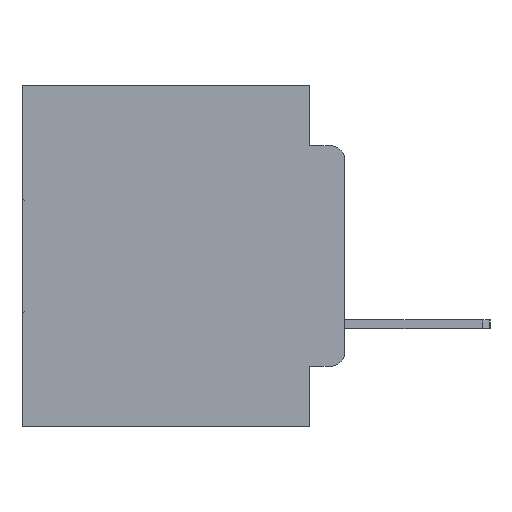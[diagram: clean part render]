
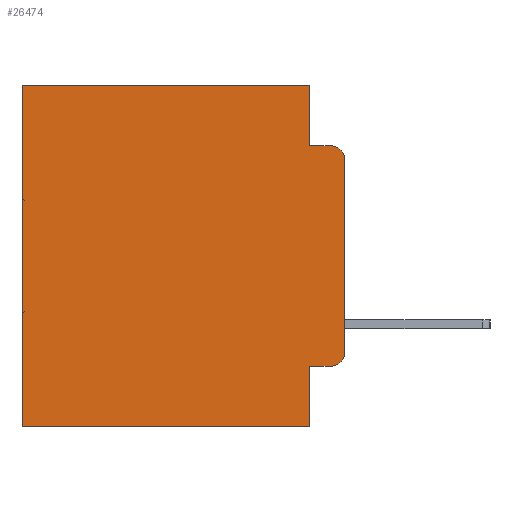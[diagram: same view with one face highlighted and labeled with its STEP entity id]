
A CAD part, left-side view. The second image highlights one B-rep face of the part: STEP entity #26474.
In plain terms, the highlighted planar face has unit normal (-1, 0, 0).
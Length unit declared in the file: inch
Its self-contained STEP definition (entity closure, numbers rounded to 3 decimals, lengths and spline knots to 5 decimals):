
#558 = FACE_OUTER_BOUND ( 'NONE', #12549, .T. ) ;
#746 = EDGE_CURVE ( 'NONE', #23154, #11562, #28423, .T. ) ;
#1446 = EDGE_CURVE ( 'NONE', #12191, #9325, #27314, .T. ) ;
#1615 = ORIENTED_EDGE ( 'NONE', *, *, #20073, .T. ) ;
#2730 = DIRECTION ( 'NONE',  ( 1., 0., 0. ) ) ;
#2898 = VECTOR ( 'NONE', #12194, 39.37008 ) ;
#3358 = CARTESIAN_POINT ( 'NONE',  ( 0.298, 0.02, -0.0885 ) ) ;
#3398 = CARTESIAN_POINT ( 'NONE',  ( 0.298, 0., -0.1085 ) ) ;
#3551 = VECTOR ( 'NONE', #27947, 39.37008 ) ;
#4354 = DIRECTION ( 'NONE',  ( 0., 1., 0. ) ) ;
#4423 = ORIENTED_EDGE ( 'NONE', *, *, #24221, .F. ) ;
#4922 = VERTEX_POINT ( 'NONE', #20242 ) ;
#4966 = ORIENTED_EDGE ( 'NONE', *, *, #13265, .T. ) ;
#5223 = CARTESIAN_POINT ( 'NONE',  ( 0.298, 0.473, 0. ) ) ;
#5248 = DIRECTION ( 'NONE',  ( 0., 0., -1. ) ) ;
#6202 = VERTEX_POINT ( 'NONE', #22765 ) ;
#6995 = EDGE_CURVE ( 'NONE', #4922, #6202, #16270, .T. ) ;
#7555 = AXIS2_PLACEMENT_3D ( 'NONE', #26868, #13041, #29163 ) ;
#7761 = CARTESIAN_POINT ( 'NONE',  ( 0.298, 0.473, -0.5 ) ) ;
#9250 = CARTESIAN_POINT ( 'NONE',  ( 0.298, 0., 0. ) ) ;
#9309 = LINE ( 'NONE', #26045, #2898 ) ;
#9325 = VERTEX_POINT ( 'NONE', #21580 ) ;
#9364 = DIRECTION ( 'NONE',  ( 0., -1., 0. ) ) ;
#9372 = ORIENTED_EDGE ( 'NONE', *, *, #11312, .T. ) ;
#9524 = AXIS2_PLACEMENT_3D ( 'NONE', #17017, #2730, #19335 ) ;
#9849 = DIRECTION ( 'NONE',  ( -1., 0., 0. ) ) ;
#9937 = AXIS2_PLACEMENT_3D ( 'NONE', #23793, #9849, #26096 ) ;
#10045 = CARTESIAN_POINT ( 'NONE',  ( 0.298, 0., 0. ) ) ;
#10566 = ORIENTED_EDGE ( 'NONE', *, *, #1446, .F. ) ;
#11142 = CARTESIAN_POINT ( 'NONE',  ( 0.298, 0.02, -0.4115 ) ) ;
#11312 = EDGE_CURVE ( 'NONE', #20638, #23154, #26828, .T. ) ;
#11315 = CARTESIAN_POINT ( 'NONE',  ( 0.298, 0.473, 0. ) ) ;
#11562 = VERTEX_POINT ( 'NONE', #7761 ) ;
#11699 = LINE ( 'NONE', #23319, #29414 ) ;
#12059 = ORIENTED_EDGE ( 'NONE', *, *, #27060, .T. ) ;
#12191 = VERTEX_POINT ( 'NONE', #3398 ) ;
#12194 = DIRECTION ( 'NONE',  ( 0., -1., 0. ) ) ;
#12410 = LINE ( 'NONE', #25455, #17934 ) ;
#12549 = EDGE_LOOP ( 'NONE', ( #10566, #12059, #21876, #4423, #9372, #22548, #27292, #24681, #1615, #4966 ) ) ;
#13041 = DIRECTION ( 'NONE',  ( -1., 0., 0. ) ) ;
#13139 = CARTESIAN_POINT ( 'NONE',  ( 0.298, 0.051, 0. ) ) ;
#13265 = EDGE_CURVE ( 'NONE', #24310, #9325, #16287, .T. ) ;
#13977 = DIRECTION ( 'NONE',  ( 0., 1., 0. ) ) ;
#14141 = CARTESIAN_POINT ( 'NONE',  ( 0.298, 0.051, 0. ) ) ;
#14335 = CARTESIAN_POINT ( 'NONE',  ( 0.298, 0.051, 0. ) ) ;
#15630 = CARTESIAN_POINT ( 'NONE',  ( 0.298, 0.051, -0.0885 ) ) ;
#16212 = VECTOR ( 'NONE', #5248, 39.37008 ) ;
#16270 = LINE ( 'NONE', #14141, #3551 ) ;
#16287 = CIRCLE ( 'NONE', #7555, 0.02 ) ;
#17017 = CARTESIAN_POINT ( 'NONE',  ( 0.298, 0., 0. ) ) ;
#17934 = VECTOR ( 'NONE', #13977, 39.37008 ) ;
#18982 = DIRECTION ( 'NONE',  ( 0., 0., -1. ) ) ;
#19335 = DIRECTION ( 'NONE',  ( 0., 0., -1. ) ) ;
#20073 = EDGE_CURVE ( 'NONE', #4922, #24310, #11699, .T. ) ;
#20148 = DIRECTION ( 'NONE',  ( 0., 0., -1. ) ) ;
#20242 = CARTESIAN_POINT ( 'NONE',  ( 0.298, 0.051, -0.4115 ) ) ;
#20638 = VERTEX_POINT ( 'NONE', #14335 ) ;
#20730 = VECTOR ( 'NONE', #4354, 39.37008 ) ;
#21187 = VECTOR ( 'NONE', #18982, 39.37008 ) ;
#21580 = CARTESIAN_POINT ( 'NONE',  ( 0.298, 0., -0.3915 ) ) ;
#21876 = ORIENTED_EDGE ( 'NONE', *, *, #22255, .F. ) ;
#22255 = EDGE_CURVE ( 'NONE', #26083, #22478, #9309, .T. ) ;
#22478 = VERTEX_POINT ( 'NONE', #3358 ) ;
#22548 = ORIENTED_EDGE ( 'NONE', *, *, #746, .T. ) ;
#22765 = CARTESIAN_POINT ( 'NONE',  ( 0.298, 0.051, -0.5 ) ) ;
#23154 = VERTEX_POINT ( 'NONE', #11315 ) ;
#23319 = CARTESIAN_POINT ( 'NONE',  ( 0.298, 0.051, -0.4115 ) ) ;
#23793 = CARTESIAN_POINT ( 'NONE',  ( 0.298, 0.02, -0.1085 ) ) ;
#23833 = EDGE_CURVE ( 'NONE', #6202, #11562, #12410, .T. ) ;
#23969 = VECTOR ( 'NONE', #20148, 39.37008 ) ;
#24221 = EDGE_CURVE ( 'NONE', #20638, #26083, #30037, .T. ) ;
#24310 = VERTEX_POINT ( 'NONE', #11142 ) ;
#24681 = ORIENTED_EDGE ( 'NONE', *, *, #6995, .F. ) ;
#25455 = CARTESIAN_POINT ( 'NONE',  ( 0.298, 0., -0.5 ) ) ;
#26045 = CARTESIAN_POINT ( 'NONE',  ( 0.298, 0.051, -0.0885 ) ) ;
#26083 = VERTEX_POINT ( 'NONE', #15630 ) ;
#26096 = DIRECTION ( 'NONE',  ( 0., 0., -1. ) ) ;
#26474 = ADVANCED_FACE ( 'NONE', ( #558 ), #28457, .F. ) ;
#26647 = CIRCLE ( 'NONE', #9937, 0.02 ) ;
#26828 = LINE ( 'NONE', #9250, #20730 ) ;
#26868 = CARTESIAN_POINT ( 'NONE',  ( 0.298, 0.02, -0.3915 ) ) ;
#27060 = EDGE_CURVE ( 'NONE', #12191, #22478, #26647, .T. ) ;
#27292 = ORIENTED_EDGE ( 'NONE', *, *, #23833, .F. ) ;
#27314 = LINE ( 'NONE', #10045, #21187 ) ;
#27947 = DIRECTION ( 'NONE',  ( 0., 0., -1. ) ) ;
#28423 = LINE ( 'NONE', #5223, #16212 ) ;
#28457 = PLANE ( 'NONE',  #9524 ) ;
#29163 = DIRECTION ( 'NONE',  ( 0., 0., -1. ) ) ;
#29414 = VECTOR ( 'NONE', #9364, 39.37008 ) ;
#30037 = LINE ( 'NONE', #13139, #23969 ) ;
